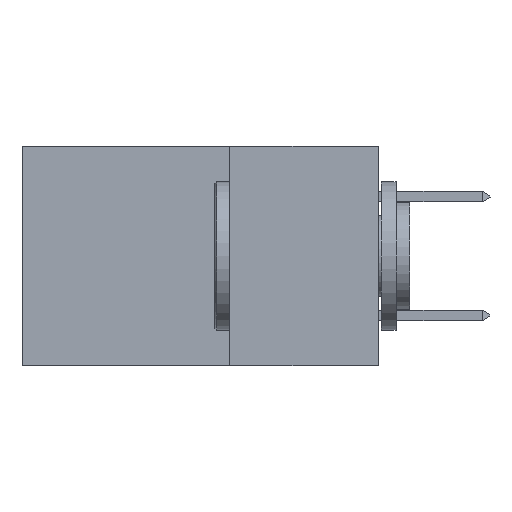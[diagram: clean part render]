
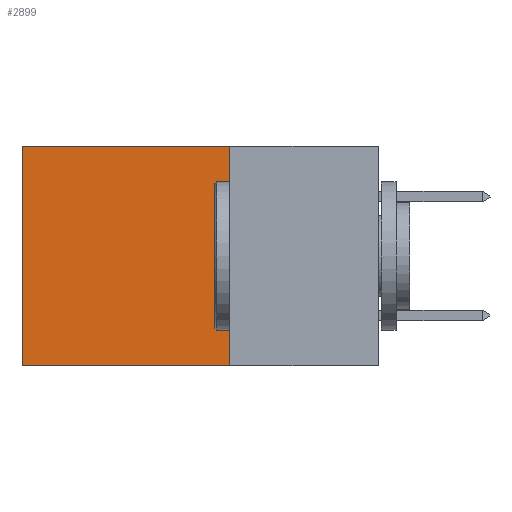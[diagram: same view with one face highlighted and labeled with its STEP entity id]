
A CAD part, left-side view. The second image highlights one B-rep face of the part: STEP entity #2899.
In plain terms, the highlighted planar face has unit normal (-1, 0, 0).
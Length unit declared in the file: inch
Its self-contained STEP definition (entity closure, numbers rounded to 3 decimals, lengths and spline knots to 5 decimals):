
#1182 = FACE_OUTER_BOUND ( 'NONE', #3126, .T. ) ;
#1732 = CARTESIAN_POINT ( 'NONE',  ( 0.298, 0.25, 0. ) ) ;
#2899 = ADVANCED_FACE ( 'NONE', ( #1182 ), #7607, .F. ) ;
#3126 = EDGE_LOOP ( 'NONE', ( #23877, #21029, #3186, #14548 ) ) ;
#3186 = ORIENTED_EDGE ( 'NONE', *, *, #16537, .F. ) ;
#3617 = CARTESIAN_POINT ( 'NONE',  ( 0.298, 0.6, 0. ) ) ;
#4420 = VERTEX_POINT ( 'NONE', #7917 ) ;
#5271 = VECTOR ( 'NONE', #14692, 39.37008 ) ;
#6359 = VECTOR ( 'NONE', #26086, 39.37008 ) ;
#6619 = VERTEX_POINT ( 'NONE', #14969 ) ;
#7607 = PLANE ( 'NONE',  #8068 ) ;
#7917 = CARTESIAN_POINT ( 'NONE',  ( 0.298, 0.6, -0.37 ) ) ;
#7951 = DIRECTION ( 'NONE',  ( 0., 0., -1. ) ) ;
#8068 = AXIS2_PLACEMENT_3D ( 'NONE', #10026, #18114, #18168 ) ;
#10026 = CARTESIAN_POINT ( 'NONE',  ( 0.298, 0.25, 0. ) ) ;
#10982 = LINE ( 'NONE', #25167, #5271 ) ;
#11262 = VECTOR ( 'NONE', #7951, 39.37008 ) ;
#11982 = CARTESIAN_POINT ( 'NONE',  ( 0.298, 0.25, -0.37 ) ) ;
#14548 = ORIENTED_EDGE ( 'NONE', *, *, #17421, .T. ) ;
#14692 = DIRECTION ( 'NONE',  ( 0., 1., 0. ) ) ;
#14969 = CARTESIAN_POINT ( 'NONE',  ( 0.298, 0.6, 0. ) ) ;
#15623 = CARTESIAN_POINT ( 'NONE',  ( 0.298, 0.25, 0. ) ) ;
#16537 = EDGE_CURVE ( 'NONE', #17753, #18863, #17774, .T. ) ;
#16950 = LINE ( 'NONE', #3617, #11262 ) ;
#17421 = EDGE_CURVE ( 'NONE', #17753, #6619, #19081, .T. ) ;
#17753 = VERTEX_POINT ( 'NONE', #1732 ) ;
#17774 = LINE ( 'NONE', #27496, #22772 ) ;
#18114 = DIRECTION ( 'NONE',  ( 1., 0., 0. ) ) ;
#18168 = DIRECTION ( 'NONE',  ( 0., 0., -1. ) ) ;
#18863 = VERTEX_POINT ( 'NONE', #11982 ) ;
#19081 = LINE ( 'NONE', #15623, #6359 ) ;
#21029 = ORIENTED_EDGE ( 'NONE', *, *, #26343, .F. ) ;
#21444 = DIRECTION ( 'NONE',  ( 0., 0., -1. ) ) ;
#22389 = EDGE_CURVE ( 'NONE', #6619, #4420, #16950, .T. ) ;
#22772 = VECTOR ( 'NONE', #21444, 39.37008 ) ;
#23877 = ORIENTED_EDGE ( 'NONE', *, *, #22389, .T. ) ;
#25167 = CARTESIAN_POINT ( 'NONE',  ( 0.298, 0.25, -0.37 ) ) ;
#26086 = DIRECTION ( 'NONE',  ( 0., 1., 0. ) ) ;
#26343 = EDGE_CURVE ( 'NONE', #18863, #4420, #10982, .T. ) ;
#27496 = CARTESIAN_POINT ( 'NONE',  ( 0.298, 0.25, 0. ) ) ;
